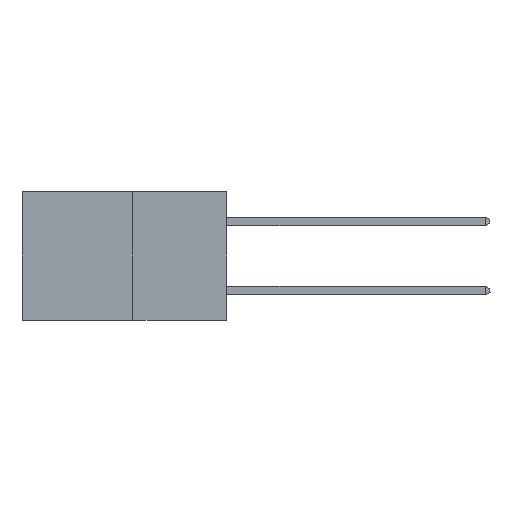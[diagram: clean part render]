
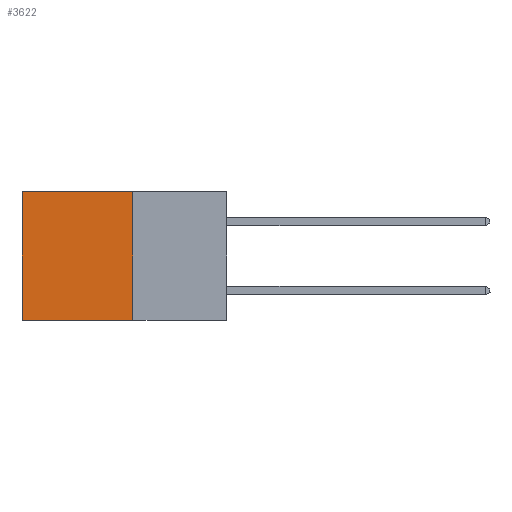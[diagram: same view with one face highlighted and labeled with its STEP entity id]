
A CAD part, left-side view. The second image highlights one B-rep face of the part: STEP entity #3622.
In plain terms, the highlighted planar face has unit normal (-1, 0, 0).
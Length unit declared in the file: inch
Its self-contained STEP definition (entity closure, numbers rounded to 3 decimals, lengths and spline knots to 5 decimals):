
#40 = DIRECTION ( 'NONE',  ( 1., 0., 0. ) ) ;
#887 = DIRECTION ( 'NONE',  ( 0., 0., -1. ) ) ;
#1268 = VECTOR ( 'NONE', #887, 39.37008 ) ;
#1461 = DIRECTION ( 'NONE',  ( 0., 1., 0. ) ) ;
#1969 = DIRECTION ( 'NONE',  ( 0., 0., -1. ) ) ;
#2109 = ORIENTED_EDGE ( 'NONE', *, *, #12068, .F. ) ;
#2188 = ORIENTED_EDGE ( 'NONE', *, *, #11379, .T. ) ;
#2332 = ORIENTED_EDGE ( 'NONE', *, *, #10066, .F. ) ;
#2487 = CARTESIAN_POINT ( 'NONE',  ( 0.277, 0.27, -0.37 ) ) ;
#2847 = VECTOR ( 'NONE', #1461, 39.37008 ) ;
#2994 = VERTEX_POINT ( 'NONE', #6621 ) ;
#3160 = CARTESIAN_POINT ( 'NONE',  ( 0.277, 0.27, -0.37 ) ) ;
#3622 = ADVANCED_FACE ( 'NONE', ( #4500 ), #10639, .F. ) ;
#4500 = FACE_OUTER_BOUND ( 'NONE', #5701, .T. ) ;
#5069 = LINE ( 'NONE', #7212, #2847 ) ;
#5701 = EDGE_LOOP ( 'NONE', ( #9019, #2109, #2332, #2188 ) ) ;
#6201 = AXIS2_PLACEMENT_3D ( 'NONE', #8300, #40, #1969 ) ;
#6621 = CARTESIAN_POINT ( 'NONE',  ( 0.277, 0.27, 0. ) ) ;
#6639 = CARTESIAN_POINT ( 'NONE',  ( 0.277, 0.59, -0.37 ) ) ;
#6720 = VERTEX_POINT ( 'NONE', #9226 ) ;
#7146 = EDGE_CURVE ( 'NONE', #6720, #7708, #11415, .T. ) ;
#7212 = CARTESIAN_POINT ( 'NONE',  ( 0.277, 0.27, 0. ) ) ;
#7480 = VECTOR ( 'NONE', #11894, 39.37008 ) ;
#7708 = VERTEX_POINT ( 'NONE', #6639 ) ;
#8149 = CARTESIAN_POINT ( 'NONE',  ( 0.277, 0.27, -0.37 ) ) ;
#8236 = DIRECTION ( 'NONE',  ( 0., 0., -1. ) ) ;
#8300 = CARTESIAN_POINT ( 'NONE',  ( 0.277, 0.27, -0.37 ) ) ;
#8491 = CARTESIAN_POINT ( 'NONE',  ( 0.277, 0.59, -0.37 ) ) ;
#9019 = ORIENTED_EDGE ( 'NONE', *, *, #7146, .T. ) ;
#9106 = VERTEX_POINT ( 'NONE', #3160 ) ;
#9226 = CARTESIAN_POINT ( 'NONE',  ( 0.277, 0.59, 0. ) ) ;
#10041 = LINE ( 'NONE', #8149, #7480 ) ;
#10066 = EDGE_CURVE ( 'NONE', #2994, #9106, #10520, .T. ) ;
#10238 = VECTOR ( 'NONE', #8236, 39.37008 ) ;
#10520 = LINE ( 'NONE', #2487, #10238 ) ;
#10639 = PLANE ( 'NONE',  #6201 ) ;
#11379 = EDGE_CURVE ( 'NONE', #2994, #6720, #5069, .T. ) ;
#11415 = LINE ( 'NONE', #8491, #1268 ) ;
#11894 = DIRECTION ( 'NONE',  ( 0., 1., 0. ) ) ;
#12068 = EDGE_CURVE ( 'NONE', #9106, #7708, #10041, .T. ) ;
